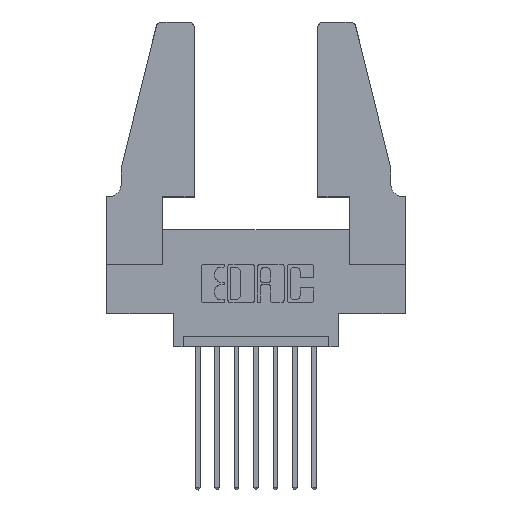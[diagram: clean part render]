
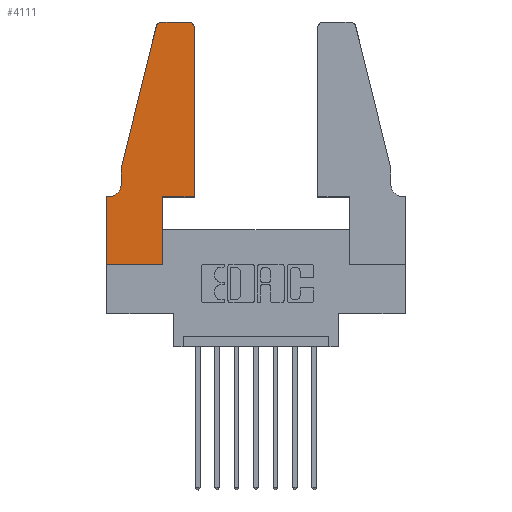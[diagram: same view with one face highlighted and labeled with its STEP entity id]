
A CAD part, top view. The second image highlights one B-rep face of the part: STEP entity #4111.
In plain terms, the highlighted planar face has unit normal (0, 0, 1).
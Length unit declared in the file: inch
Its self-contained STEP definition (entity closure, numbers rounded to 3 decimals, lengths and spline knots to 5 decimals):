
#116 = CARTESIAN_POINT ( 'NONE',  ( 0., 0.35, 0.37 ) ) ;
#260 = CARTESIAN_POINT ( 'NONE',  ( 0.2865, 0.35, 0.37 ) ) ;
#315 = EDGE_CURVE ( 'NONE', #12253, #4663, #2343, .T. ) ;
#887 = DIRECTION ( 'NONE',  ( 0., -1., 0. ) ) ;
#890 = EDGE_LOOP ( 'NONE', ( #8215, #3061, #4345, #6106, #10043, #11904, #11482, #2771, #2989, #4309, #1840, #1446 ) ) ;
#985 = VECTOR ( 'NONE', #887, 39.37008 ) ;
#1067 = EDGE_CURVE ( 'NONE', #2959, #6406, #12004, .T. ) ;
#1253 = CARTESIAN_POINT ( 'NONE',  ( 0.284, 1.22, 0.37 ) ) ;
#1367 = EDGE_CURVE ( 'NONE', #5631, #7260, #9482, .T. ) ;
#1368 = VECTOR ( 'NONE', #11563, 39.37008 ) ;
#1446 = ORIENTED_EDGE ( 'NONE', *, *, #2492, .T. ) ;
#1840 = ORIENTED_EDGE ( 'NONE', *, *, #315, .T. ) ;
#1857 = DIRECTION ( 'NONE',  ( 1., 0., 0. ) ) ;
#1867 = EDGE_CURVE ( 'NONE', #2868, #9506, #4995, .T. ) ;
#1910 = CARTESIAN_POINT ( 'NONE',  ( 0.0755, 0.5, 0.37 ) ) ;
#2324 = EDGE_CURVE ( 'NONE', #2444, #8459, #10931, .T. ) ;
#2343 = LINE ( 'NONE', #3177, #3692 ) ;
#2444 = VERTEX_POINT ( 'NONE', #6568 ) ;
#2492 = EDGE_CURVE ( 'NONE', #4663, #5631, #4114, .T. ) ;
#2686 = VECTOR ( 'NONE', #7770, 39.37008 ) ;
#2767 = CARTESIAN_POINT ( 'NONE',  ( 0.4205, 1.22, 0.37 ) ) ;
#2771 = ORIENTED_EDGE ( 'NONE', *, *, #11907, .T. ) ;
#2838 = DIRECTION ( 'NONE',  ( 1., 0., 0. ) ) ;
#2868 = VERTEX_POINT ( 'NONE', #4410 ) ;
#2959 = VERTEX_POINT ( 'NONE', #6446 ) ;
#2978 = VECTOR ( 'NONE', #9942, 39.37008 ) ;
#2989 = ORIENTED_EDGE ( 'NONE', *, *, #5397, .T. ) ;
#3056 = AXIS2_PLACEMENT_3D ( 'NONE', #1253, #7923, #8875 ) ;
#3061 = ORIENTED_EDGE ( 'NONE', *, *, #5674, .T. ) ;
#3072 = CARTESIAN_POINT ( 'NONE',  ( 0.0055, 0.42, 0.37 ) ) ;
#3177 = CARTESIAN_POINT ( 'NONE',  ( 0.4505, 0.35, 0.37 ) ) ;
#3592 = LINE ( 'NONE', #260, #2686 ) ;
#3692 = VECTOR ( 'NONE', #10790, 39.37008 ) ;
#3746 = DIRECTION ( 'NONE',  ( 0., 0., 1. ) ) ;
#3758 = DIRECTION ( 'NONE',  ( -0.239, -0.971, 0. ) ) ;
#4111 = ADVANCED_FACE ( 'NONE', ( #11342 ), #11448, .T. ) ;
#4114 = CIRCLE ( 'NONE', #4389, 0.03 ) ;
#4309 = ORIENTED_EDGE ( 'NONE', *, *, #11031, .T. ) ;
#4341 = CARTESIAN_POINT ( 'NONE',  ( 0.0755, 0.5, 0.37 ) ) ;
#4345 = ORIENTED_EDGE ( 'NONE', *, *, #2324, .T. ) ;
#4389 = AXIS2_PLACEMENT_3D ( 'NONE', #2767, #3746, #1857 ) ;
#4410 = CARTESIAN_POINT ( 'NONE',  ( 0., 0.35, 0.37 ) ) ;
#4615 = CARTESIAN_POINT ( 'NONE',  ( 0.2605, 1.25, 0.37 ) ) ;
#4663 = VERTEX_POINT ( 'NONE', #4790 ) ;
#4790 = CARTESIAN_POINT ( 'NONE',  ( 0.4505, 1.22, 0.37 ) ) ;
#4995 = LINE ( 'NONE', #11324, #985 ) ;
#5217 = CARTESIAN_POINT ( 'NONE',  ( 0.0755, 0.5, 0.37 ) ) ;
#5269 = VECTOR ( 'NONE', #6345, 39.37008 ) ;
#5397 = EDGE_CURVE ( 'NONE', #12184, #11470, #3592, .T. ) ;
#5631 = VERTEX_POINT ( 'NONE', #8647 ) ;
#5674 = EDGE_CURVE ( 'NONE', #7260, #2444, #11930, .T. ) ;
#5860 = CARTESIAN_POINT ( 'NONE',  ( 0.2865, 0., 0.37 ) ) ;
#5936 = LINE ( 'NONE', #5217, #2978 ) ;
#6106 = ORIENTED_EDGE ( 'NONE', *, *, #6721, .T. ) ;
#6345 = DIRECTION ( 'NONE',  ( -1., 0., 0. ) ) ;
#6406 = VERTEX_POINT ( 'NONE', #12284 ) ;
#6424 = CARTESIAN_POINT ( 'NONE',  ( 0.4505, 0.35, 0.37 ) ) ;
#6446 = CARTESIAN_POINT ( 'NONE',  ( 0.0755, 0.42, 0.37 ) ) ;
#6564 = LINE ( 'NONE', #7627, #10438 ) ;
#6568 = CARTESIAN_POINT ( 'NONE',  ( 0.25487, 1.22718, 0.37 ) ) ;
#6609 = AXIS2_PLACEMENT_3D ( 'NONE', #3072, #10733, #7910 ) ;
#6721 = EDGE_CURVE ( 'NONE', #8459, #2959, #5936, .T. ) ;
#6862 = CARTESIAN_POINT ( 'NONE',  ( 0.4505, 0.35, 0.37 ) ) ;
#7028 = AXIS2_PLACEMENT_3D ( 'NONE', #116, #8677, #2838 ) ;
#7260 = VERTEX_POINT ( 'NONE', #7496 ) ;
#7496 = CARTESIAN_POINT ( 'NONE',  ( 0.284, 1.25, 0.37 ) ) ;
#7515 = VECTOR ( 'NONE', #3758, 39.37008 ) ;
#7627 = CARTESIAN_POINT ( 'NONE',  ( 0., 0., 0.37 ) ) ;
#7770 = DIRECTION ( 'NONE',  ( 0., 1., 0. ) ) ;
#7910 = DIRECTION ( 'NONE',  ( -1., 0., 0. ) ) ;
#7923 = DIRECTION ( 'NONE',  ( 0., 0., 1. ) ) ;
#7946 = EDGE_CURVE ( 'NONE', #6406, #2868, #11586, .T. ) ;
#8215 = ORIENTED_EDGE ( 'NONE', *, *, #1367, .T. ) ;
#8449 = VECTOR ( 'NONE', #10843, 39.37008 ) ;
#8459 = VERTEX_POINT ( 'NONE', #4341 ) ;
#8647 = CARTESIAN_POINT ( 'NONE',  ( 0.4205, 1.25, 0.37 ) ) ;
#8677 = DIRECTION ( 'NONE',  ( 0., 0., 1. ) ) ;
#8875 = DIRECTION ( 'NONE',  ( 1., 0., 0. ) ) ;
#9370 = DIRECTION ( 'NONE',  ( 1., 0., 0. ) ) ;
#9482 = LINE ( 'NONE', #4615, #5269 ) ;
#9506 = VERTEX_POINT ( 'NONE', #11882 ) ;
#9942 = DIRECTION ( 'NONE',  ( 0., -1., 0. ) ) ;
#10009 = CARTESIAN_POINT ( 'NONE',  ( 0.0755, 0.35, 0.37 ) ) ;
#10043 = ORIENTED_EDGE ( 'NONE', *, *, #1067, .T. ) ;
#10438 = VECTOR ( 'NONE', #9370, 39.37008 ) ;
#10733 = DIRECTION ( 'NONE',  ( 0., 0., -1. ) ) ;
#10790 = DIRECTION ( 'NONE',  ( 0., 1., 0. ) ) ;
#10843 = DIRECTION ( 'NONE',  ( -1., 0., 0. ) ) ;
#10931 = LINE ( 'NONE', #1910, #7515 ) ;
#11031 = EDGE_CURVE ( 'NONE', #11470, #12253, #11662, .T. ) ;
#11324 = CARTESIAN_POINT ( 'NONE',  ( 0., 0., 0.37 ) ) ;
#11342 = FACE_OUTER_BOUND ( 'NONE', #890, .T. ) ;
#11448 = PLANE ( 'NONE',  #7028 ) ;
#11470 = VERTEX_POINT ( 'NONE', #12176 ) ;
#11482 = ORIENTED_EDGE ( 'NONE', *, *, #1867, .T. ) ;
#11563 = DIRECTION ( 'NONE',  ( 1., 0., 0. ) ) ;
#11586 = LINE ( 'NONE', #10009, #8449 ) ;
#11662 = LINE ( 'NONE', #6862, #1368 ) ;
#11882 = CARTESIAN_POINT ( 'NONE',  ( 0., 0., 0.37 ) ) ;
#11904 = ORIENTED_EDGE ( 'NONE', *, *, #7946, .T. ) ;
#11907 = EDGE_CURVE ( 'NONE', #9506, #12184, #6564, .T. ) ;
#11930 = CIRCLE ( 'NONE', #3056, 0.03 ) ;
#12004 = CIRCLE ( 'NONE', #6609, 0.07 ) ;
#12176 = CARTESIAN_POINT ( 'NONE',  ( 0.2865, 0.35, 0.37 ) ) ;
#12184 = VERTEX_POINT ( 'NONE', #5860 ) ;
#12253 = VERTEX_POINT ( 'NONE', #6424 ) ;
#12284 = CARTESIAN_POINT ( 'NONE',  ( 0.0055, 0.35, 0.37 ) ) ;
